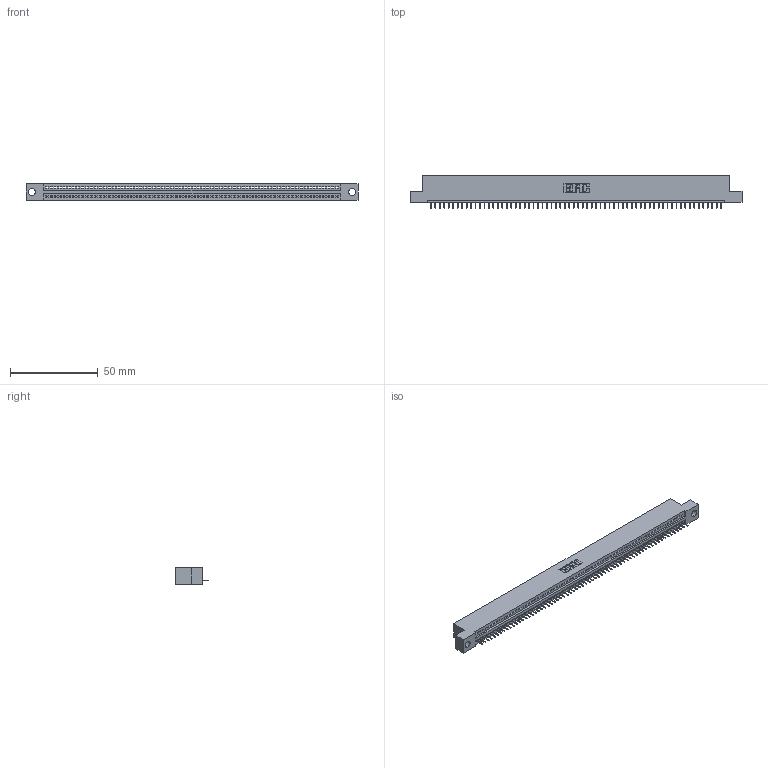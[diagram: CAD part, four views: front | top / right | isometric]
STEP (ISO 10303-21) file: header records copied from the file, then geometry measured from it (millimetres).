
FILE_DESCRIPTION (( 'STEP AP203' ), '1' );
FILE_NAME ('395-066-525-104.STEP', '2020-09-25T01:11:02', ( '' ), ( '' ), 'SwSTEP 2.0', 'SolidWorks 2020', '' );
FILE_SCHEMA (( 'CONFIG_CONTROL_DESIGN' ));
Length unit declared in the file: inch
Products named in the file (3): 345 Part_Flush Mounting Lugs - 0.156 Dia-TH; 345-292-001_345-293-125; 395-066-525-104
Assembly tree (67 placements, depth 2):
  395-066-525-104
    345 Part_Flush Mounting Lugs - 0.156 Dia-TH
    345-292-001_345-293-125  x66
Bounding box: 188.85 x 18.72 x 9.4 mm (x, y, z)
Volume: 17776.3 mm3; surface area: 22859.5 mm2
Topology: 67 solids, 67 shells, 4218 faces, 12221 edges, 7882 vertices
Faces by surface type: plane 3116, cylinder 1102
Entity records: 46519 total; most frequent: ORIENTED_EDGE 8062, CARTESIAN_POINT 8062, DIRECTION 7007, EDGE_CURVE 4031, LINE 3639, VECTOR 3639, VERTEX_POINT 2682, AXIS2_PLACEMENT_3D 1684
